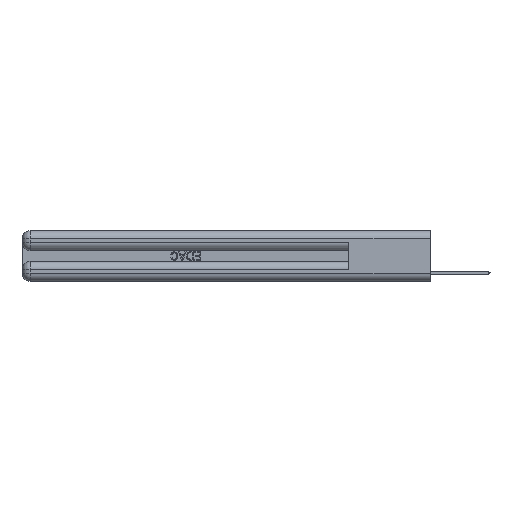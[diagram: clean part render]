
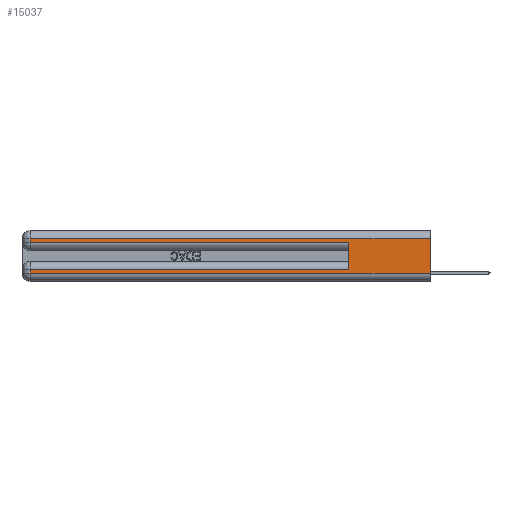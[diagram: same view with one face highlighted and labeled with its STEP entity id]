
A CAD part, left-side view. The second image highlights one B-rep face of the part: STEP entity #15037.
In plain terms, the highlighted planar face has unit normal (-1, 0, 0).
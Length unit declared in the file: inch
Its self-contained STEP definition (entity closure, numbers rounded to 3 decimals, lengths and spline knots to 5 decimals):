
#305 = CARTESIAN_POINT ( 'NONE',  ( 0., 0.6, 0.085 ) ) ;
#800 = ORIENTED_EDGE ( 'NONE', *, *, #18526, .T. ) ;
#1067 = CARTESIAN_POINT ( 'NONE',  ( 0., 0., 0.085 ) ) ;
#1186 = DIRECTION ( 'NONE',  ( 0., 1., 0. ) ) ;
#1191 = VERTEX_POINT ( 'NONE', #26717 ) ;
#1520 = VECTOR ( 'NONE', #15705, 39.37008 ) ;
#2002 = CARTESIAN_POINT ( 'NONE',  ( 0., 0.6, 0.285 ) ) ;
#2187 = ORIENTED_EDGE ( 'NONE', *, *, #30392, .F. ) ;
#2265 = LINE ( 'NONE', #7959, #4266 ) ;
#2802 = ORIENTED_EDGE ( 'NONE', *, *, #10801, .T. ) ;
#2822 = DIRECTION ( 'NONE',  ( 0., 0., -1. ) ) ;
#2879 = VECTOR ( 'NONE', #1186, 39.37008 ) ;
#2999 = VERTEX_POINT ( 'NONE', #5931 ) ;
#3980 = VECTOR ( 'NONE', #14925, 39.37008 ) ;
#4266 = VECTOR ( 'NONE', #2822, 39.37008 ) ;
#4308 = VECTOR ( 'NONE', #4530, 39.37008 ) ;
#4530 = DIRECTION ( 'NONE',  ( 0., 1., 0. ) ) ;
#4849 = ORIENTED_EDGE ( 'NONE', *, *, #25921, .F. ) ;
#5931 = CARTESIAN_POINT ( 'NONE',  ( 0., 2.94, 0.31 ) ) ;
#5980 = CARTESIAN_POINT ( 'NONE',  ( 0., 0., 0.37 ) ) ;
#6763 = VECTOR ( 'NONE', #8504, 39.37008 ) ;
#7227 = ORIENTED_EDGE ( 'NONE', *, *, #10425, .T. ) ;
#7606 = CARTESIAN_POINT ( 'NONE',  ( 0., 2.94, 0.37 ) ) ;
#7959 = CARTESIAN_POINT ( 'NONE',  ( 0., 0., 0.37 ) ) ;
#8504 = DIRECTION ( 'NONE',  ( 0., -1., 0. ) ) ;
#9556 = ORIENTED_EDGE ( 'NONE', *, *, #20837, .T. ) ;
#9568 = ORIENTED_EDGE ( 'NONE', *, *, #22228, .T. ) ;
#10425 = EDGE_CURVE ( 'NONE', #21912, #1191, #15558, .T. ) ;
#10676 = VERTEX_POINT ( 'NONE', #2002 ) ;
#10801 = EDGE_CURVE ( 'NONE', #2999, #28976, #14312, .T. ) ;
#10892 = VERTEX_POINT ( 'NONE', #305 ) ;
#11125 = CARTESIAN_POINT ( 'NONE',  ( 0., 2.94, 0.06 ) ) ;
#11991 = CARTESIAN_POINT ( 'NONE',  ( 0., 2.94, 0.085 ) ) ;
#14312 = LINE ( 'NONE', #7606, #23551 ) ;
#14576 = CARTESIAN_POINT ( 'NONE',  ( 0., 0., 0.31 ) ) ;
#14925 = DIRECTION ( 'NONE',  ( 0., 0., 1. ) ) ;
#14972 = FACE_OUTER_BOUND ( 'NONE', #27331, .T. ) ;
#15037 = ADVANCED_FACE ( 'NONE', ( #14972 ), #21195, .F. ) ;
#15150 = LINE ( 'NONE', #31063, #1520 ) ;
#15178 = LINE ( 'NONE', #30043, #3980 ) ;
#15249 = VERTEX_POINT ( 'NONE', #11991 ) ;
#15558 = LINE ( 'NONE', #29090, #6763 ) ;
#15705 = DIRECTION ( 'NONE',  ( 0., -1., 0. ) ) ;
#16749 = DIRECTION ( 'NONE',  ( 0., 0., -1. ) ) ;
#17696 = LINE ( 'NONE', #1067, #2879 ) ;
#18526 = EDGE_CURVE ( 'NONE', #15249, #21912, #20398, .T. ) ;
#18837 = DIRECTION ( 'NONE',  ( 1., 0., 0. ) ) ;
#19256 = VERTEX_POINT ( 'NONE', #22462 ) ;
#20398 = LINE ( 'NONE', #26793, #31614 ) ;
#20837 = EDGE_CURVE ( 'NONE', #28976, #10676, #15150, .T. ) ;
#21195 = PLANE ( 'NONE',  #25628 ) ;
#21912 = VERTEX_POINT ( 'NONE', #11125 ) ;
#22228 = EDGE_CURVE ( 'NONE', #19256, #2999, #23506, .T. ) ;
#22462 = CARTESIAN_POINT ( 'NONE',  ( 0., 0., 0.31 ) ) ;
#23506 = LINE ( 'NONE', #14576, #4308 ) ;
#23551 = VECTOR ( 'NONE', #30432, 39.37008 ) ;
#23758 = DIRECTION ( 'NONE',  ( 0., 0., -1. ) ) ;
#24562 = CARTESIAN_POINT ( 'NONE',  ( 0., 2.94, 0.285 ) ) ;
#25628 = AXIS2_PLACEMENT_3D ( 'NONE', #5980, #18837, #23758 ) ;
#25921 = EDGE_CURVE ( 'NONE', #19256, #1191, #2265, .T. ) ;
#26717 = CARTESIAN_POINT ( 'NONE',  ( 0., 0., 0.06 ) ) ;
#26793 = CARTESIAN_POINT ( 'NONE',  ( 0., 2.94, 0.37 ) ) ;
#27331 = EDGE_LOOP ( 'NONE', ( #4849, #9568, #2802, #9556, #2187, #29798, #800, #7227 ) ) ;
#28729 = EDGE_CURVE ( 'NONE', #10892, #15249, #17696, .T. ) ;
#28976 = VERTEX_POINT ( 'NONE', #24562 ) ;
#29090 = CARTESIAN_POINT ( 'NONE',  ( 0., 0., 0.06 ) ) ;
#29798 = ORIENTED_EDGE ( 'NONE', *, *, #28729, .T. ) ;
#30043 = CARTESIAN_POINT ( 'NONE',  ( 0., 0.6, 0.145 ) ) ;
#30392 = EDGE_CURVE ( 'NONE', #10892, #10676, #15178, .T. ) ;
#30432 = DIRECTION ( 'NONE',  ( 0., 0., -1. ) ) ;
#31063 = CARTESIAN_POINT ( 'NONE',  ( 0., 0., 0.285 ) ) ;
#31614 = VECTOR ( 'NONE', #16749, 39.37008 ) ;
